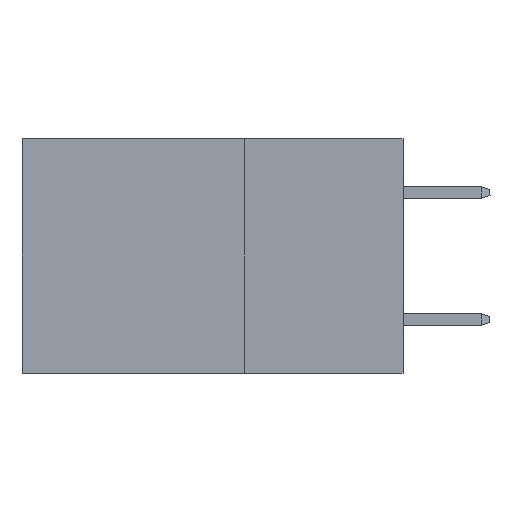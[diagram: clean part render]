
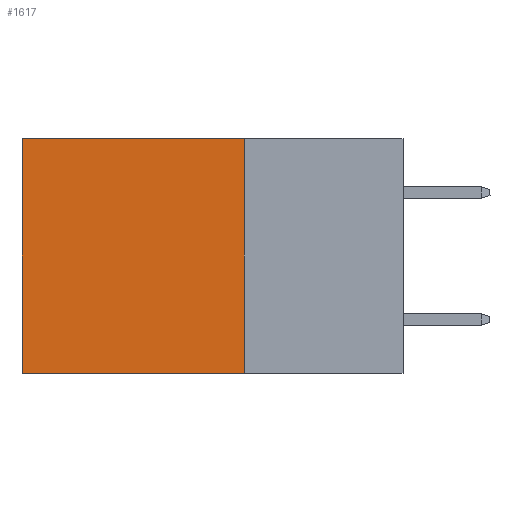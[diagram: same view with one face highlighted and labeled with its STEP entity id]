
A CAD part, left-side view. The second image highlights one B-rep face of the part: STEP entity #1617.
In plain terms, the highlighted planar face has unit normal (-1, 0, 0).
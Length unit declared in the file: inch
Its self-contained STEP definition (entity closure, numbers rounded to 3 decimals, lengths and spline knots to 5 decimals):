
#348 = EDGE_CURVE ( 'NONE', #7391, #3728, #15296, .T. ) ;
#513 = CARTESIAN_POINT ( 'NONE',  ( 0.2875, 0.25, -0.37 ) ) ;
#959 = DIRECTION ( 'NONE',  ( 1., 0., 0. ) ) ;
#1617 = ADVANCED_FACE ( 'NONE', ( #14676 ), #16088, .F. ) ;
#1901 = CARTESIAN_POINT ( 'NONE',  ( 0.2875, 0.25, 0. ) ) ;
#2069 = CARTESIAN_POINT ( 'NONE',  ( 0.2875, 0.6, -0.37 ) ) ;
#2600 = CARTESIAN_POINT ( 'NONE',  ( 0.2875, 0.25, 0. ) ) ;
#3131 = LINE ( 'NONE', #8178, #10671 ) ;
#3381 = CARTESIAN_POINT ( 'NONE',  ( 0.2875, 0.25, 0. ) ) ;
#3728 = VERTEX_POINT ( 'NONE', #513 ) ;
#4585 = CARTESIAN_POINT ( 'NONE',  ( 0.2875, 0.25, -0.37 ) ) ;
#4644 = CARTESIAN_POINT ( 'NONE',  ( 0.2875, 0.25, 0. ) ) ;
#4947 = EDGE_CURVE ( 'NONE', #3728, #15540, #9633, .T. ) ;
#5824 = LINE ( 'NONE', #3381, #14008 ) ;
#6241 = EDGE_CURVE ( 'NONE', #7391, #14865, #5824, .T. ) ;
#6755 = ORIENTED_EDGE ( 'NONE', *, *, #4947, .F. ) ;
#7056 = DIRECTION ( 'NONE',  ( 0., 1., 0. ) ) ;
#7288 = DIRECTION ( 'NONE',  ( 0., 1., 0. ) ) ;
#7391 = VERTEX_POINT ( 'NONE', #4644 ) ;
#8178 = CARTESIAN_POINT ( 'NONE',  ( 0.2875, 0.6, 0. ) ) ;
#8504 = VECTOR ( 'NONE', #7288, 39.37008 ) ;
#8841 = VECTOR ( 'NONE', #9244, 39.37008 ) ;
#8867 = EDGE_LOOP ( 'NONE', ( #15339, #6755, #14978, #14431 ) ) ;
#9115 = CARTESIAN_POINT ( 'NONE',  ( 0.2875, 0.6, 0. ) ) ;
#9244 = DIRECTION ( 'NONE',  ( 0., 0., -1. ) ) ;
#9279 = EDGE_CURVE ( 'NONE', #14865, #15540, #3131, .T. ) ;
#9488 = DIRECTION ( 'NONE',  ( 0., 0., -1. ) ) ;
#9614 = DIRECTION ( 'NONE',  ( 0., 0., -1. ) ) ;
#9633 = LINE ( 'NONE', #4585, #8504 ) ;
#9979 = AXIS2_PLACEMENT_3D ( 'NONE', #2600, #959, #9614 ) ;
#10671 = VECTOR ( 'NONE', #9488, 39.37008 ) ;
#14008 = VECTOR ( 'NONE', #7056, 39.37008 ) ;
#14431 = ORIENTED_EDGE ( 'NONE', *, *, #6241, .T. ) ;
#14676 = FACE_OUTER_BOUND ( 'NONE', #8867, .T. ) ;
#14865 = VERTEX_POINT ( 'NONE', #9115 ) ;
#14978 = ORIENTED_EDGE ( 'NONE', *, *, #348, .F. ) ;
#15296 = LINE ( 'NONE', #1901, #8841 ) ;
#15339 = ORIENTED_EDGE ( 'NONE', *, *, #9279, .T. ) ;
#15540 = VERTEX_POINT ( 'NONE', #2069 ) ;
#16088 = PLANE ( 'NONE',  #9979 ) ;
